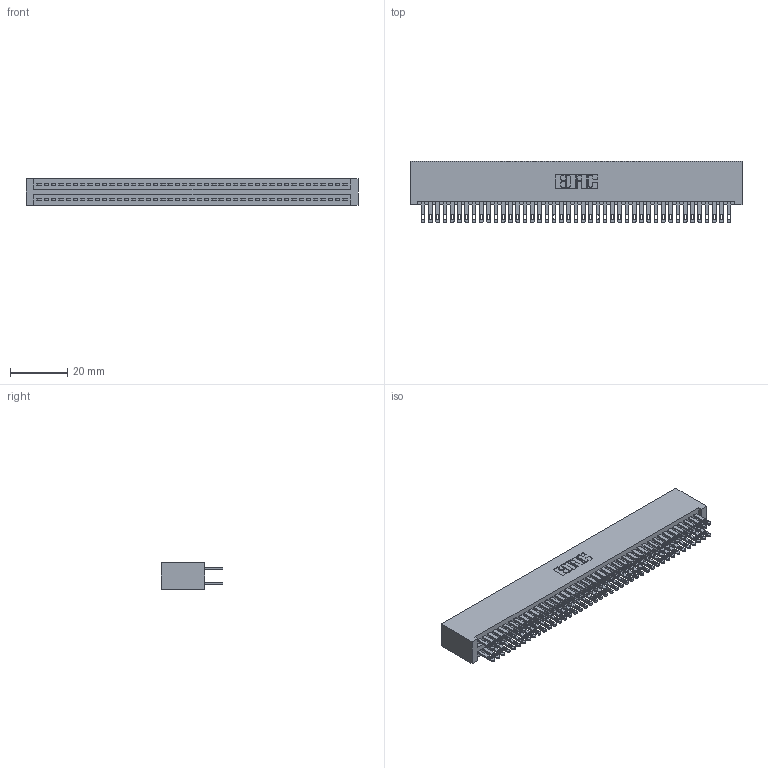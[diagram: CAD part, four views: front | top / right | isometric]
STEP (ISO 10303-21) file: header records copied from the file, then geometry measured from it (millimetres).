
FILE_DESCRIPTION (( 'STEP AP203' ), '1' );
FILE_NAME ('345-086-500-201.STEP', '2018-10-04T03:55:41', ( '' ), ( '' ), 'SwSTEP 2.0', 'SolidWorks 2016', '' );
FILE_SCHEMA (( 'CONFIG_CONTROL_DESIGN' ));
Length unit declared in the file: inch
Products named in the file (3): 345 Part_No Mounting Lugs; 345-292-001_345-293-100; 345-086-500-201
Assembly tree (87 placements, depth 2):
  345-086-500-201
    345 Part_No Mounting Lugs
    345-292-001_345-293-100  x86
Bounding box: 115.82 x 21.51 x 9.4 mm (x, y, z)
Volume: 12139.3 mm3; surface area: 19143.6 mm2
Topology: 87 solids, 87 shells, 4074 faces, 12443 edges, 8294 vertices
Faces by surface type: plane 2398, cylinder 1676
Entity records: 33257 total; most frequent: CARTESIAN_POINT 5572, ORIENTED_EDGE 5506, DIRECTION 4909, EDGE_CURVE 2753, LINE 2453, VECTOR 2453, VERTEX_POINT 1834, AXIS2_PLACEMENT_3D 1228
